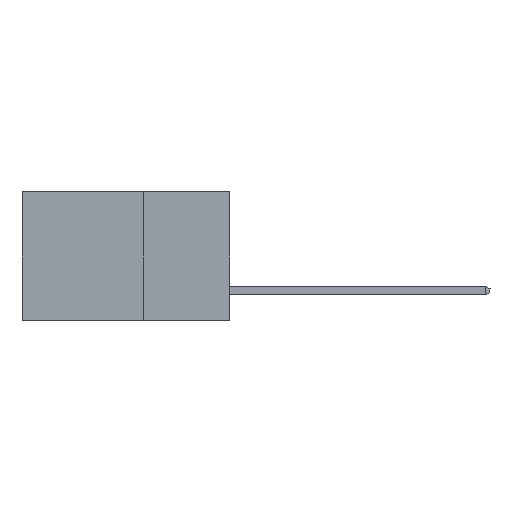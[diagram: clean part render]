
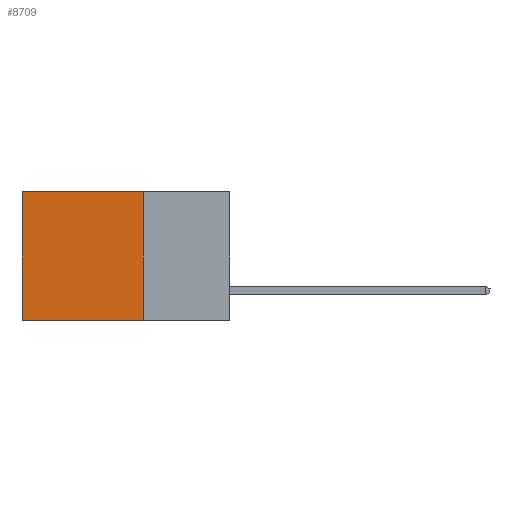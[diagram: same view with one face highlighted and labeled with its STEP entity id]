
A CAD part, left-side view. The second image highlights one B-rep face of the part: STEP entity #8709.
In plain terms, the highlighted planar face has unit normal (-1, 0, 0).
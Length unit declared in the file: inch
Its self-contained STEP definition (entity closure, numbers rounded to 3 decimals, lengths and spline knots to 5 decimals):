
#5 = VECTOR ( 'NONE', #19758, 39.37008 ) ;
#521 = EDGE_CURVE ( 'NONE', #15715, #13817, #14549, .T. ) ;
#672 = DIRECTION ( 'NONE',  ( 1., 0., 0. ) ) ;
#1049 = AXIS2_PLACEMENT_3D ( 'NONE', #15514, #672, #8671 ) ;
#1303 = LINE ( 'NONE', #16369, #2020 ) ;
#2020 = VECTOR ( 'NONE', #19586, 39.37008 ) ;
#2957 = VECTOR ( 'NONE', #12898, 39.37008 ) ;
#3798 = EDGE_CURVE ( 'NONE', #6488, #5837, #6467, .T. ) ;
#4089 = ORIENTED_EDGE ( 'NONE', *, *, #521, .T. ) ;
#5661 = ORIENTED_EDGE ( 'NONE', *, *, #5798, .F. ) ;
#5798 = EDGE_CURVE ( 'NONE', #15715, #6488, #1303, .T. ) ;
#5837 = VERTEX_POINT ( 'NONE', #16432 ) ;
#6467 = LINE ( 'NONE', #9709, #11551 ) ;
#6488 = VERTEX_POINT ( 'NONE', #18325 ) ;
#7322 = FACE_OUTER_BOUND ( 'NONE', #16765, .T. ) ;
#7379 = CARTESIAN_POINT ( 'NONE',  ( 0.2615, 0.6, 0. ) ) ;
#7907 = CARTESIAN_POINT ( 'NONE',  ( 0.2615, 0.25, 0. ) ) ;
#8039 = DIRECTION ( 'NONE',  ( 0., 1., 0. ) ) ;
#8426 = ORIENTED_EDGE ( 'NONE', *, *, #3798, .F. ) ;
#8671 = DIRECTION ( 'NONE',  ( 0., 0., -1. ) ) ;
#8709 = ADVANCED_FACE ( 'NONE', ( #7322 ), #20810, .F. ) ;
#9117 = ORIENTED_EDGE ( 'NONE', *, *, #13993, .T. ) ;
#9709 = CARTESIAN_POINT ( 'NONE',  ( 0.2615, 0.25, -0.37 ) ) ;
#10442 = LINE ( 'NONE', #11760, #5 ) ;
#11551 = VECTOR ( 'NONE', #8039, 39.37008 ) ;
#11760 = CARTESIAN_POINT ( 'NONE',  ( 0.2615, 0.6, -0.37 ) ) ;
#12898 = DIRECTION ( 'NONE',  ( 0., 1., 0. ) ) ;
#13100 = CARTESIAN_POINT ( 'NONE',  ( 0.2615, 0.25, 0. ) ) ;
#13817 = VERTEX_POINT ( 'NONE', #7379 ) ;
#13993 = EDGE_CURVE ( 'NONE', #13817, #5837, #10442, .T. ) ;
#14549 = LINE ( 'NONE', #7907, #2957 ) ;
#15514 = CARTESIAN_POINT ( 'NONE',  ( 0.2615, 0.25, -0.37 ) ) ;
#15715 = VERTEX_POINT ( 'NONE', #13100 ) ;
#16369 = CARTESIAN_POINT ( 'NONE',  ( 0.2615, 0.25, -0.37 ) ) ;
#16432 = CARTESIAN_POINT ( 'NONE',  ( 0.2615, 0.6, -0.37 ) ) ;
#16765 = EDGE_LOOP ( 'NONE', ( #9117, #8426, #5661, #4089 ) ) ;
#18325 = CARTESIAN_POINT ( 'NONE',  ( 0.2615, 0.25, -0.37 ) ) ;
#19586 = DIRECTION ( 'NONE',  ( 0., 0., -1. ) ) ;
#19758 = DIRECTION ( 'NONE',  ( 0., 0., -1. ) ) ;
#20810 = PLANE ( 'NONE',  #1049 ) ;
